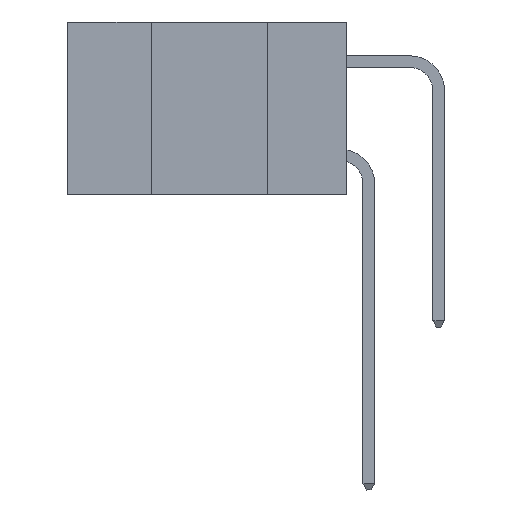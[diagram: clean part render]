
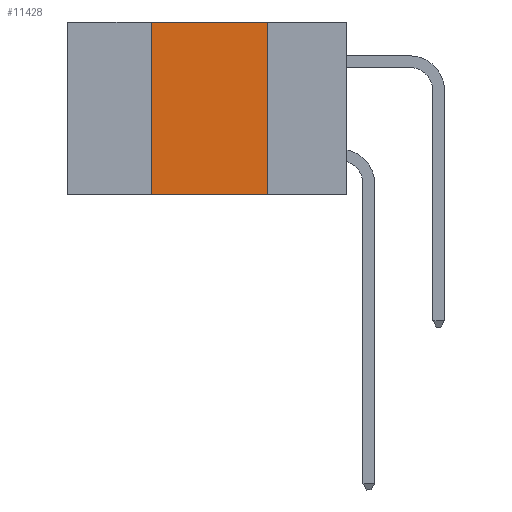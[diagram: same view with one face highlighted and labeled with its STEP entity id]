
A CAD part, left-side view. The second image highlights one B-rep face of the part: STEP entity #11428.
In plain terms, the highlighted planar face has unit normal (-1, 0, 0).
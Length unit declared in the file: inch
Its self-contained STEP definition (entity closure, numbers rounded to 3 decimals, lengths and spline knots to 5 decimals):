
#554 = CARTESIAN_POINT ( 'NONE',  ( 0., 0.17, 0. ) ) ;
#658 = CARTESIAN_POINT ( 'NONE',  ( 0., 0.6, 0. ) ) ;
#1011 = VECTOR ( 'NONE', #2279, 39.37008 ) ;
#1592 = EDGE_CURVE ( 'NONE', #4241, #7295, #6383, .T. ) ;
#2004 = ORIENTED_EDGE ( 'NONE', *, *, #8428, .T. ) ;
#2279 = DIRECTION ( 'NONE',  ( 0., 0., -1. ) ) ;
#3036 = CARTESIAN_POINT ( 'NONE',  ( 0., 0.6, 0. ) ) ;
#3174 = VECTOR ( 'NONE', #8767, 39.37008 ) ;
#3297 = ORIENTED_EDGE ( 'NONE', *, *, #1592, .F. ) ;
#4066 = PLANE ( 'NONE',  #10849 ) ;
#4132 = CARTESIAN_POINT ( 'NONE',  ( 0., 0.17, 0. ) ) ;
#4241 = VERTEX_POINT ( 'NONE', #17380 ) ;
#4635 = LINE ( 'NONE', #16437, #9444 ) ;
#5831 = DIRECTION ( 'NONE',  ( 0., 0., -1. ) ) ;
#6383 = LINE ( 'NONE', #3036, #10425 ) ;
#6490 = DIRECTION ( 'NONE',  ( 0., -1., 0. ) ) ;
#7046 = ORIENTED_EDGE ( 'NONE', *, *, #15098, .F. ) ;
#7295 = VERTEX_POINT ( 'NONE', #4132 ) ;
#7740 = LINE ( 'NONE', #20867, #3174 ) ;
#8428 = EDGE_CURVE ( 'NONE', #16573, #14159, #7740, .T. ) ;
#8767 = DIRECTION ( 'NONE',  ( 0., -1., 0. ) ) ;
#8788 = CARTESIAN_POINT ( 'NONE',  ( 0., 0.17, -0.37 ) ) ;
#8837 = EDGE_LOOP ( 'NONE', ( #13688, #3297, #7046, #2004 ) ) ;
#9444 = VECTOR ( 'NONE', #11274, 39.37008 ) ;
#10425 = VECTOR ( 'NONE', #6490, 39.37008 ) ;
#10849 = AXIS2_PLACEMENT_3D ( 'NONE', #658, #16204, #5831 ) ;
#11274 = DIRECTION ( 'NONE',  ( 0., 0., 1. ) ) ;
#11428 = ADVANCED_FACE ( 'NONE', ( #14389 ), #4066, .F. ) ;
#12518 = CARTESIAN_POINT ( 'NONE',  ( 0., 0.42, -0.37 ) ) ;
#13688 = ORIENTED_EDGE ( 'NONE', *, *, #21152, .F. ) ;
#14159 = VERTEX_POINT ( 'NONE', #8788 ) ;
#14389 = FACE_OUTER_BOUND ( 'NONE', #8837, .T. ) ;
#15098 = EDGE_CURVE ( 'NONE', #16573, #4241, #4635, .T. ) ;
#16204 = DIRECTION ( 'NONE',  ( 1., 0., 0. ) ) ;
#16437 = CARTESIAN_POINT ( 'NONE',  ( 0., 0.42, 0. ) ) ;
#16573 = VERTEX_POINT ( 'NONE', #12518 ) ;
#17380 = CARTESIAN_POINT ( 'NONE',  ( 0., 0.42, 0. ) ) ;
#19344 = LINE ( 'NONE', #554, #1011 ) ;
#20867 = CARTESIAN_POINT ( 'NONE',  ( 0., 0.6, -0.37 ) ) ;
#21152 = EDGE_CURVE ( 'NONE', #7295, #14159, #19344, .T. ) ;
